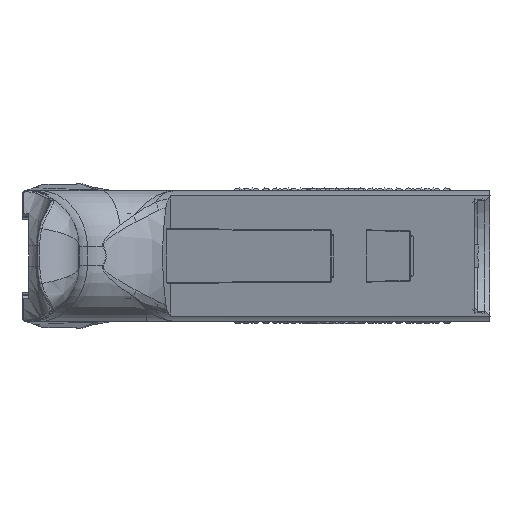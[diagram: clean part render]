
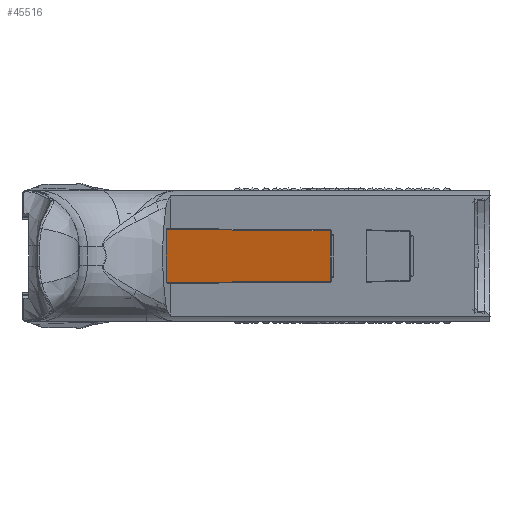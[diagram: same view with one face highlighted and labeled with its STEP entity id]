
A CAD part, left-side view. The second image highlights one B-rep face of the part: STEP entity #45516.
In plain terms, the highlighted planar face has unit normal (-0.951, 0.309, 0).
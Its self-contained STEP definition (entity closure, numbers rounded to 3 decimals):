
#1638 = DIRECTION ( 'NONE',  ( 0., 0., 1. ) ) ;
#4348 = VERTEX_POINT ( 'NONE', #102057 ) ;
#5545 = CARTESIAN_POINT ( 'NONE',  ( -61.056, 19.838, 0. ) ) ;
#12921 = CARTESIAN_POINT ( 'NONE',  ( -73.586, -18.725, -25.314 ) ) ;
#13756 = VECTOR ( 'NONE', #66686, 1000. ) ;
#15968 = ORIENTED_EDGE ( 'NONE', *, *, #126365, .T. ) ;
#15998 = DIRECTION ( 'NONE',  ( -0.309, -0.951, 0. ) ) ;
#16362 = EDGE_CURVE ( 'NONE', #133012, #78602, #144123, .T. ) ;
#25407 = EDGE_CURVE ( 'NONE', #57567, #133012, #130452, .T. ) ;
#35907 = ORIENTED_EDGE ( 'NONE', *, *, #25407, .T. ) ;
#35963 = LINE ( 'NONE', #90353, #101449 ) ;
#40912 = DIRECTION ( 'NONE',  ( -0.309, -0.951, 0.006 ) ) ;
#41981 = EDGE_CURVE ( 'NONE', #4348, #55323, #35963, .T. ) ;
#45235 = DIRECTION ( 'NONE',  ( -0.951, 0.309, 0. ) ) ;
#45516 = ADVANCED_FACE ( 'NONE', ( #79021 ), #92821, .T. ) ;
#51305 = LINE ( 'NONE', #91832, #144766 ) ;
#55323 = VERTEX_POINT ( 'NONE', #78126 ) ;
#57567 = VERTEX_POINT ( 'NONE', #162306 ) ;
#57589 = CARTESIAN_POINT ( 'NONE',  ( -61.812, 17.51, -25.35 ) ) ;
#66686 = DIRECTION ( 'NONE',  ( 0.309, 0.951, 0.006 ) ) ;
#78126 = CARTESIAN_POINT ( 'NONE',  ( -73.586, -18.725, -25.113 ) ) ;
#78602 = VERTEX_POINT ( 'NONE', #57589 ) ;
#79021 = FACE_OUTER_BOUND ( 'NONE', #86928, .T. ) ;
#82689 = DIRECTION ( 'NONE',  ( 0., 0., -1. ) ) ;
#86928 = EDGE_LOOP ( 'NONE', ( #135676, #15968, #168558, #96634, #35907 ) ) ;
#89109 = VECTOR ( 'NONE', #82689, 1000. ) ;
#90353 = CARTESIAN_POINT ( 'NONE',  ( -71.278, -11.623, -32.673 ) ) ;
#91832 = CARTESIAN_POINT ( 'NONE',  ( -73.586, -18.724, -25.114 ) ) ;
#92821 = PLANE ( 'NONE',  #154195 ) ;
#94066 = EDGE_CURVE ( 'NONE', #55323, #57567, #131075, .T. ) ;
#96634 = ORIENTED_EDGE ( 'NONE', *, *, #94066, .T. ) ;
#100191 = VECTOR ( 'NONE', #1638, 1000. ) ;
#101449 = VECTOR ( 'NONE', #102500, 1000. ) ;
#102057 = CARTESIAN_POINT ( 'NONE',  ( -73.586, -18.724, -25.114 ) ) ;
#102500 = DIRECTION ( 'NONE',  ( -0.217, -0.668, 0.711 ) ) ;
#103829 = CARTESIAN_POINT ( 'NONE',  ( -61.812, 17.511, -13.65 ) ) ;
#126365 = EDGE_CURVE ( 'NONE', #78602, #4348, #51305, .T. ) ;
#130452 = LINE ( 'NONE', #103829, #13756 ) ;
#131075 = LINE ( 'NONE', #12921, #100191 ) ;
#133012 = VERTEX_POINT ( 'NONE', #155349 ) ;
#135233 = CARTESIAN_POINT ( 'NONE',  ( -61.812, 17.51, -25.55 ) ) ;
#135676 = ORIENTED_EDGE ( 'NONE', *, *, #16362, .T. ) ;
#144123 = LINE ( 'NONE', #135233, #89109 ) ;
#144766 = VECTOR ( 'NONE', #40912, 1000. ) ;
#154195 = AXIS2_PLACEMENT_3D ( 'NONE', #5545, #45235, #15998 ) ;
#155349 = CARTESIAN_POINT ( 'NONE',  ( -61.812, 17.51, -13.65 ) ) ;
#162306 = CARTESIAN_POINT ( 'NONE',  ( -73.586, -18.725, -13.886 ) ) ;
#168558 = ORIENTED_EDGE ( 'NONE', *, *, #41981, .T. ) ;
